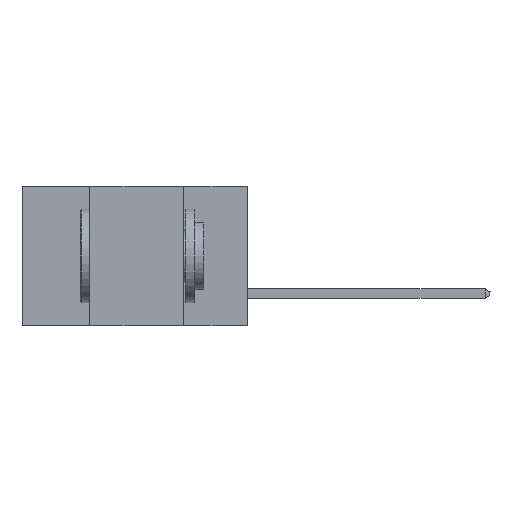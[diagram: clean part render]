
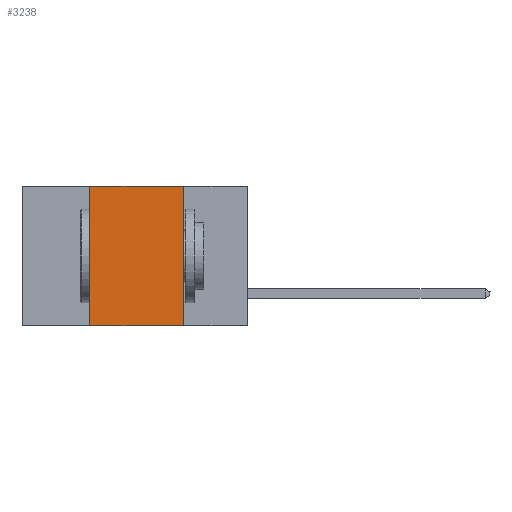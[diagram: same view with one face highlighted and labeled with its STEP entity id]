
A CAD part, left-side view. The second image highlights one B-rep face of the part: STEP entity #3238.
In plain terms, the highlighted planar face has unit normal (-1, 0, 0).
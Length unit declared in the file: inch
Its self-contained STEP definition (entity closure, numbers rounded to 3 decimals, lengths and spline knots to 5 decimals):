
#11 = CARTESIAN_POINT ( 'NONE',  ( 0., 0.17, -0.37 ) ) ;
#133 = DIRECTION ( 'NONE',  ( 0., 0., -1. ) ) ;
#1070 = VECTOR ( 'NONE', #3298, 39.37008 ) ;
#1357 = EDGE_CURVE ( 'NONE', #3465, #12363, #12210, .T. ) ;
#1435 = FACE_OUTER_BOUND ( 'NONE', #4274, .T. ) ;
#1436 = AXIS2_PLACEMENT_3D ( 'NONE', #6782, #10146, #133 ) ;
#1560 = LINE ( 'NONE', #7260, #8716 ) ;
#1736 = ORIENTED_EDGE ( 'NONE', *, *, #1357, .F. ) ;
#1923 = CARTESIAN_POINT ( 'NONE',  ( 0., 0.17, -0.37 ) ) ;
#2165 = EDGE_CURVE ( 'NONE', #9962, #11943, #10488, .T. ) ;
#2321 = VECTOR ( 'NONE', #6268, 39.37008 ) ;
#3180 = CARTESIAN_POINT ( 'NONE',  ( 0., 0.42, 0. ) ) ;
#3238 = ADVANCED_FACE ( 'NONE', ( #1435 ), #5619, .F. ) ;
#3298 = DIRECTION ( 'NONE',  ( 0., -1., 0. ) ) ;
#3465 = VERTEX_POINT ( 'NONE', #13214 ) ;
#3807 = DIRECTION ( 'NONE',  ( 0., -1., 0. ) ) ;
#4274 = EDGE_LOOP ( 'NONE', ( #1736, #6410, #7479, #10109 ) ) ;
#5582 = EDGE_CURVE ( 'NONE', #11943, #3465, #1560, .T. ) ;
#5619 = PLANE ( 'NONE',  #1436 ) ;
#6268 = DIRECTION ( 'NONE',  ( 0., 0., 1. ) ) ;
#6410 = ORIENTED_EDGE ( 'NONE', *, *, #5582, .F. ) ;
#6591 = LINE ( 'NONE', #11040, #1070 ) ;
#6782 = CARTESIAN_POINT ( 'NONE',  ( 0., 0.6, 0. ) ) ;
#7173 = VECTOR ( 'NONE', #10818, 39.37008 ) ;
#7260 = CARTESIAN_POINT ( 'NONE',  ( 0., 0.6, 0. ) ) ;
#7479 = ORIENTED_EDGE ( 'NONE', *, *, #2165, .F. ) ;
#8317 = CARTESIAN_POINT ( 'NONE',  ( 0., 0.42, -0.37 ) ) ;
#8716 = VECTOR ( 'NONE', #3807, 39.37008 ) ;
#9962 = VERTEX_POINT ( 'NONE', #13667 ) ;
#10109 = ORIENTED_EDGE ( 'NONE', *, *, #10662, .T. ) ;
#10146 = DIRECTION ( 'NONE',  ( 1., 0., 0. ) ) ;
#10488 = LINE ( 'NONE', #8317, #2321 ) ;
#10662 = EDGE_CURVE ( 'NONE', #9962, #12363, #6591, .T. ) ;
#10818 = DIRECTION ( 'NONE',  ( 0., 0., -1. ) ) ;
#11040 = CARTESIAN_POINT ( 'NONE',  ( 0., 0.6, -0.37 ) ) ;
#11943 = VERTEX_POINT ( 'NONE', #3180 ) ;
#12210 = LINE ( 'NONE', #11, #7173 ) ;
#12363 = VERTEX_POINT ( 'NONE', #1923 ) ;
#13214 = CARTESIAN_POINT ( 'NONE',  ( 0., 0.17, 0. ) ) ;
#13667 = CARTESIAN_POINT ( 'NONE',  ( 0., 0.42, -0.37 ) ) ;
